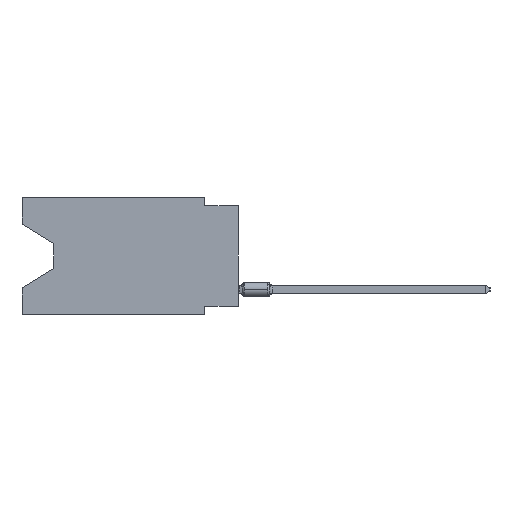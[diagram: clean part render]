
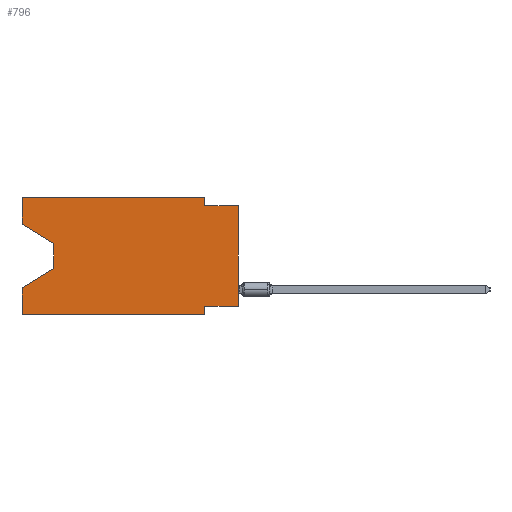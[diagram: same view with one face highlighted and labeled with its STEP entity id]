
A CAD part, left-side view. The second image highlights one B-rep face of the part: STEP entity #796.
In plain terms, the highlighted planar face has unit normal (-1, 0, 0).
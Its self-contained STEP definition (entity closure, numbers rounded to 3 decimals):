
#523 = CARTESIAN_POINT ( 'NONE',  ( 0., 16.383, -6.852 ) ) ;
#710 = EDGE_CURVE ( 'NONE', #39935, #5436, #38809, .T. ) ;
#796 = ADVANCED_FACE ( 'NONE', ( #43432 ), #25468, .F. ) ;
#1727 = VECTOR ( 'NONE', #50368, 1000. ) ;
#2018 = ORIENTED_EDGE ( 'NONE', *, *, #30802, .F. ) ;
#3173 = EDGE_CURVE ( 'NONE', #5436, #30191, #20700, .T. ) ;
#3276 = CARTESIAN_POINT ( 'NONE',  ( 0., 2.54, -8.255 ) ) ;
#3702 = EDGE_CURVE ( 'NONE', #4242, #51190, #38212, .T. ) ;
#3949 = ORIENTED_EDGE ( 'NONE', *, *, #38089, .T. ) ;
#4159 = VECTOR ( 'NONE', #54755, 1000. ) ;
#4242 = VERTEX_POINT ( 'NONE', #9949 ) ;
#4640 = LINE ( 'NONE', #28349, #1727 ) ;
#4794 = EDGE_CURVE ( 'NONE', #57177, #30191, #40878, .T. ) ;
#5436 = VERTEX_POINT ( 'NONE', #55523 ) ;
#6538 = CARTESIAN_POINT ( 'NONE',  ( 0., 16.383, -2.038 ) ) ;
#7218 = VECTOR ( 'NONE', #10630, 1000. ) ;
#7515 = DIRECTION ( 'NONE',  ( 0., 0., 1. ) ) ;
#7772 = ORIENTED_EDGE ( 'NONE', *, *, #710, .T. ) ;
#8035 = ORIENTED_EDGE ( 'NONE', *, *, #9086, .T. ) ;
#8105 = DIRECTION ( 'NONE',  ( 0., 0., -1. ) ) ;
#8416 = CARTESIAN_POINT ( 'NONE',  ( 0., 2.54, -8.89 ) ) ;
#8434 = VECTOR ( 'NONE', #41183, 1000. ) ;
#9086 = EDGE_CURVE ( 'NONE', #57177, #9380, #56086, .T. ) ;
#9165 = CARTESIAN_POINT ( 'NONE',  ( 0., 0., -0.635 ) ) ;
#9205 = DIRECTION ( 'NONE',  ( 0., 0., -1. ) ) ;
#9380 = VERTEX_POINT ( 'NONE', #8416 ) ;
#9949 = CARTESIAN_POINT ( 'NONE',  ( 0., 0., -8.255 ) ) ;
#10584 = LINE ( 'NONE', #6538, #46581 ) ;
#10630 = DIRECTION ( 'NONE',  ( 0., 1., 0. ) ) ;
#11360 = VERTEX_POINT ( 'NONE', #53800 ) ;
#11573 = ORIENTED_EDGE ( 'NONE', *, *, #32333, .F. ) ;
#12124 = CARTESIAN_POINT ( 'NONE',  ( 0., 0., 0. ) ) ;
#14646 = LINE ( 'NONE', #49704, #21612 ) ;
#16755 = ORIENTED_EDGE ( 'NONE', *, *, #49090, .F. ) ;
#16968 = DIRECTION ( 'NONE',  ( 0., -1., 0. ) ) ;
#19297 = DIRECTION ( 'NONE',  ( 0., -0.855, -0.519 ) ) ;
#19337 = LINE ( 'NONE', #32929, #7218 ) ;
#19732 = VECTOR ( 'NONE', #7515, 1000. ) ;
#20415 = ORIENTED_EDGE ( 'NONE', *, *, #22137, .F. ) ;
#20700 = LINE ( 'NONE', #24768, #21550 ) ;
#21003 = EDGE_LOOP ( 'NONE', ( #3949, #7772, #27343, #24540, #8035, #11573, #16755, #27794, #20415, #46351, #2018, #21557 ) ) ;
#21172 = CARTESIAN_POINT ( 'NONE',  ( 0., 2.54, -8.89 ) ) ;
#21410 = DIRECTION ( 'NONE',  ( 1., 0., 0. ) ) ;
#21550 = VECTOR ( 'NONE', #47354, 1000. ) ;
#21557 = ORIENTED_EDGE ( 'NONE', *, *, #49747, .F. ) ;
#21612 = VECTOR ( 'NONE', #28261, 1000. ) ;
#22137 = EDGE_CURVE ( 'NONE', #49878, #51190, #52027, .T. ) ;
#22604 = CARTESIAN_POINT ( 'NONE',  ( 0., 16.383, -2.038 ) ) ;
#23787 = VECTOR ( 'NONE', #42759, 1000. ) ;
#24540 = ORIENTED_EDGE ( 'NONE', *, *, #4794, .F. ) ;
#24768 = CARTESIAN_POINT ( 'NONE',  ( 0., 13.97, -5.385 ) ) ;
#25468 = PLANE ( 'NONE',  #52775 ) ;
#27343 = ORIENTED_EDGE ( 'NONE', *, *, #3173, .T. ) ;
#27794 = ORIENTED_EDGE ( 'NONE', *, *, #3702, .T. ) ;
#28261 = DIRECTION ( 'NONE',  ( 0., 0., -1. ) ) ;
#28349 = CARTESIAN_POINT ( 'NONE',  ( 0., 16.383, 0. ) ) ;
#30191 = VERTEX_POINT ( 'NONE', #523 ) ;
#30802 = EDGE_CURVE ( 'NONE', #45436, #11360, #4640, .T. ) ;
#31531 = VECTOR ( 'NONE', #8105, 1000. ) ;
#31874 = CARTESIAN_POINT ( 'NONE',  ( 0., 0., -0.635 ) ) ;
#32181 = CARTESIAN_POINT ( 'NONE',  ( 0., 16.383, 0. ) ) ;
#32333 = EDGE_CURVE ( 'NONE', #32609, #9380, #53221, .T. ) ;
#32609 = VERTEX_POINT ( 'NONE', #3276 ) ;
#32929 = CARTESIAN_POINT ( 'NONE',  ( 0., 0., -8.255 ) ) ;
#33799 = CARTESIAN_POINT ( 'NONE',  ( 0., 13.97, -3.505 ) ) ;
#36848 = CARTESIAN_POINT ( 'NONE',  ( 0., 16.383, 0. ) ) ;
#38089 = EDGE_CURVE ( 'NONE', #56436, #39935, #10584, .T. ) ;
#38090 = EDGE_CURVE ( 'NONE', #11360, #49878, #14646, .T. ) ;
#38212 = LINE ( 'NONE', #12124, #19732 ) ;
#38809 = LINE ( 'NONE', #56741, #31531 ) ;
#38835 = CARTESIAN_POINT ( 'NONE',  ( 0., 2.54, -0.635 ) ) ;
#38947 = VECTOR ( 'NONE', #16968, 1000. ) ;
#39935 = VERTEX_POINT ( 'NONE', #33799 ) ;
#40878 = LINE ( 'NONE', #32181, #4159 ) ;
#41183 = DIRECTION ( 'NONE',  ( 0., 0., 1. ) ) ;
#41533 = VECTOR ( 'NONE', #9205, 1000. ) ;
#42068 = CARTESIAN_POINT ( 'NONE',  ( 0., 16.383, 0. ) ) ;
#42759 = DIRECTION ( 'NONE',  ( 0., -1., 0. ) ) ;
#43432 = FACE_OUTER_BOUND ( 'NONE', #21003, .T. ) ;
#45436 = VERTEX_POINT ( 'NONE', #42068 ) ;
#46351 = ORIENTED_EDGE ( 'NONE', *, *, #38090, .F. ) ;
#46581 = VECTOR ( 'NONE', #19297, 1000. ) ;
#47354 = DIRECTION ( 'NONE',  ( 0., 0.855, -0.519 ) ) ;
#49090 = EDGE_CURVE ( 'NONE', #4242, #32609, #19337, .T. ) ;
#49704 = CARTESIAN_POINT ( 'NONE',  ( 0., 2.54, 0. ) ) ;
#49747 = EDGE_CURVE ( 'NONE', #56436, #45436, #50161, .T. ) ;
#49878 = VERTEX_POINT ( 'NONE', #38835 ) ;
#50161 = LINE ( 'NONE', #36848, #8434 ) ;
#50368 = DIRECTION ( 'NONE',  ( 0., -1., 0. ) ) ;
#50887 = CARTESIAN_POINT ( 'NONE',  ( 0., 16.383, -8.89 ) ) ;
#51190 = VERTEX_POINT ( 'NONE', #31874 ) ;
#52027 = LINE ( 'NONE', #9165, #38947 ) ;
#52107 = DIRECTION ( 'NONE',  ( 0., 0., -1. ) ) ;
#52775 = AXIS2_PLACEMENT_3D ( 'NONE', #56462, #21410, #52107 ) ;
#53221 = LINE ( 'NONE', #21172, #41533 ) ;
#53800 = CARTESIAN_POINT ( 'NONE',  ( 0., 2.54, 0. ) ) ;
#54755 = DIRECTION ( 'NONE',  ( 0., 0., 1. ) ) ;
#55523 = CARTESIAN_POINT ( 'NONE',  ( 0., 13.97, -5.385 ) ) ;
#56086 = LINE ( 'NONE', #50887, #23787 ) ;
#56436 = VERTEX_POINT ( 'NONE', #22604 ) ;
#56462 = CARTESIAN_POINT ( 'NONE',  ( 0., 16.383, 0. ) ) ;
#56741 = CARTESIAN_POINT ( 'NONE',  ( 0., 13.97, -3.505 ) ) ;
#57173 = CARTESIAN_POINT ( 'NONE',  ( 0., 16.383, -8.89 ) ) ;
#57177 = VERTEX_POINT ( 'NONE', #57173 ) ;
